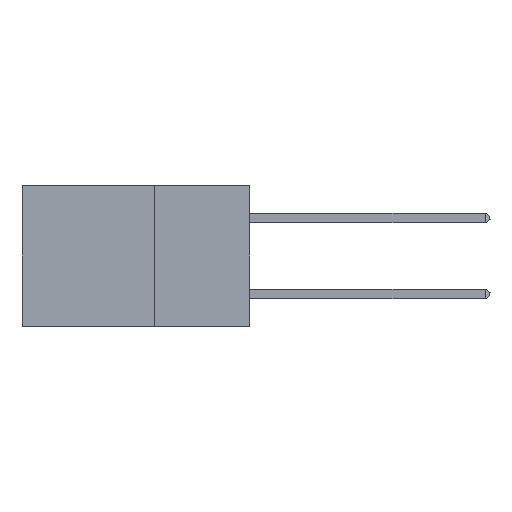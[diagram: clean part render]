
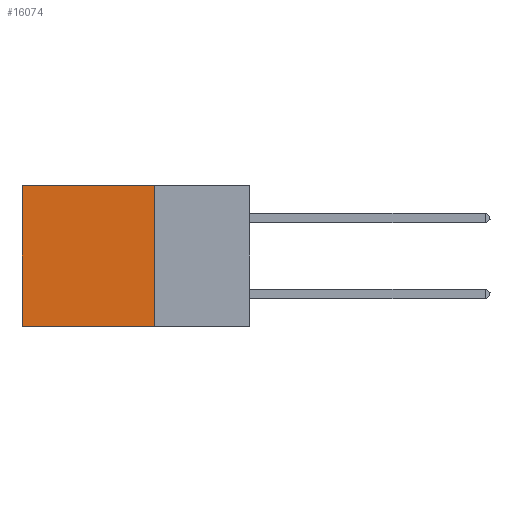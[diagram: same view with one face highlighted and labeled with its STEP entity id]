
A CAD part, left-side view. The second image highlights one B-rep face of the part: STEP entity #16074.
In plain terms, the highlighted planar face has unit normal (-1, 0, 0).
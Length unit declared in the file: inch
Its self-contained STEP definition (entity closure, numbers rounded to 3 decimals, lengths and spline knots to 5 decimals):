
#1714 = LINE ( 'NONE', #13969, #11938 ) ;
#2014 = CARTESIAN_POINT ( 'NONE',  ( 0.2875, 0.6, 0. ) ) ;
#2369 = LINE ( 'NONE', #3632, #5594 ) ;
#2435 = ORIENTED_EDGE ( 'NONE', *, *, #8265, .T. ) ;
#2577 = ORIENTED_EDGE ( 'NONE', *, *, #4003, .F. ) ;
#3005 = DIRECTION ( 'NONE',  ( 1., 0., 0. ) ) ;
#3350 = VERTEX_POINT ( 'NONE', #8889 ) ;
#3632 = CARTESIAN_POINT ( 'NONE',  ( 0.2875, 0.25, -0.37 ) ) ;
#4003 = EDGE_CURVE ( 'NONE', #6149, #9938, #1714, .T. ) ;
#4371 = EDGE_CURVE ( 'NONE', #6149, #11064, #7007, .T. ) ;
#4968 = DIRECTION ( 'NONE',  ( 0., 1., 0. ) ) ;
#5010 = VECTOR ( 'NONE', #9709, 39.37008 ) ;
#5424 = LINE ( 'NONE', #8387, #5010 ) ;
#5594 = VECTOR ( 'NONE', #4968, 39.37008 ) ;
#6145 = DIRECTION ( 'NONE',  ( 0., 0., -1. ) ) ;
#6149 = VERTEX_POINT ( 'NONE', #10787 ) ;
#7007 = LINE ( 'NONE', #14983, #13939 ) ;
#7741 = AXIS2_PLACEMENT_3D ( 'NONE', #10965, #3005, #12287 ) ;
#8265 = EDGE_CURVE ( 'NONE', #11064, #3350, #5424, .T. ) ;
#8387 = CARTESIAN_POINT ( 'NONE',  ( 0.2875, 0.6, 0. ) ) ;
#8889 = CARTESIAN_POINT ( 'NONE',  ( 0.2875, 0.6, -0.37 ) ) ;
#8991 = CARTESIAN_POINT ( 'NONE',  ( 0.2875, 0.25, -0.37 ) ) ;
#9379 = EDGE_CURVE ( 'NONE', #9938, #3350, #2369, .T. ) ;
#9569 = FACE_OUTER_BOUND ( 'NONE', #13084, .T. ) ;
#9709 = DIRECTION ( 'NONE',  ( 0., 0., -1. ) ) ;
#9938 = VERTEX_POINT ( 'NONE', #8991 ) ;
#10787 = CARTESIAN_POINT ( 'NONE',  ( 0.2875, 0.25, 0. ) ) ;
#10909 = PLANE ( 'NONE',  #7741 ) ;
#10965 = CARTESIAN_POINT ( 'NONE',  ( 0.2875, 0.25, 0. ) ) ;
#11064 = VERTEX_POINT ( 'NONE', #2014 ) ;
#11470 = ORIENTED_EDGE ( 'NONE', *, *, #9379, .F. ) ;
#11938 = VECTOR ( 'NONE', #6145, 39.37008 ) ;
#12287 = DIRECTION ( 'NONE',  ( 0., 0., -1. ) ) ;
#12867 = ORIENTED_EDGE ( 'NONE', *, *, #4371, .T. ) ;
#13084 = EDGE_LOOP ( 'NONE', ( #2435, #11470, #2577, #12867 ) ) ;
#13939 = VECTOR ( 'NONE', #16316, 39.37008 ) ;
#13969 = CARTESIAN_POINT ( 'NONE',  ( 0.2875, 0.25, 0. ) ) ;
#14983 = CARTESIAN_POINT ( 'NONE',  ( 0.2875, 0.25, 0. ) ) ;
#16074 = ADVANCED_FACE ( 'NONE', ( #9569 ), #10909, .F. ) ;
#16316 = DIRECTION ( 'NONE',  ( 0., 1., 0. ) ) ;
